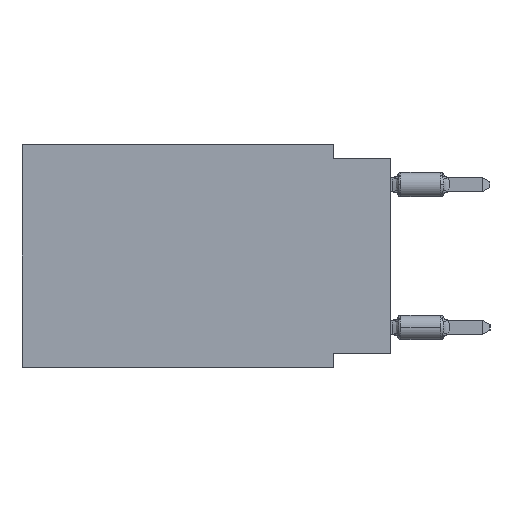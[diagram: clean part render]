
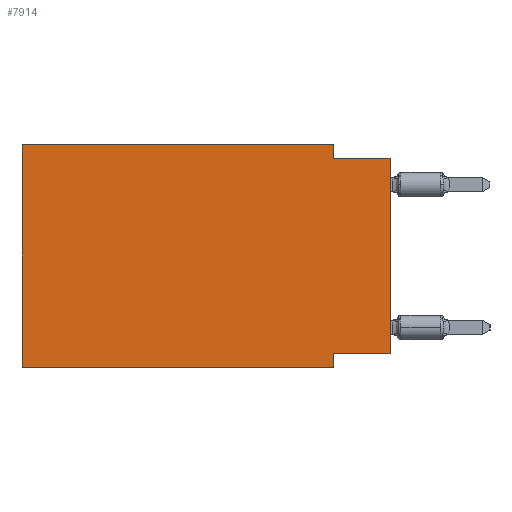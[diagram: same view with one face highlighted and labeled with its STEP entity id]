
A CAD part, left-side view. The second image highlights one B-rep face of the part: STEP entity #7914.
In plain terms, the highlighted planar face has unit normal (-1, 0, 0).
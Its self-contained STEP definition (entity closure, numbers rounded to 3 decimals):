
#79 = VECTOR ( 'NONE', #2542, 1000. ) ;
#182 = CARTESIAN_POINT ( 'NONE',  ( 0., 16.383, -9.906 ) ) ;
#345 = FACE_OUTER_BOUND ( 'NONE', #1507, .T. ) ;
#1161 = DIRECTION ( 'NONE',  ( 0., 1., 0. ) ) ;
#1223 = LINE ( 'NONE', #20597, #79 ) ;
#1426 = AXIS2_PLACEMENT_3D ( 'NONE', #5745, #12348, #20137 ) ;
#1507 = EDGE_LOOP ( 'NONE', ( #10673, #5341, #10723, #15838, #16441, #10533, #19143, #2085 ) ) ;
#1753 = DIRECTION ( 'NONE',  ( 0., -1., 0. ) ) ;
#1975 = VECTOR ( 'NONE', #2917, 1000. ) ;
#2085 = ORIENTED_EDGE ( 'NONE', *, *, #8417, .F. ) ;
#2102 = CARTESIAN_POINT ( 'NONE',  ( 0., 0., 0. ) ) ;
#2542 = DIRECTION ( 'NONE',  ( 0., 0., -1. ) ) ;
#2917 = DIRECTION ( 'NONE',  ( 0., -1., 0. ) ) ;
#3406 = EDGE_CURVE ( 'NONE', #12749, #7236, #16147, .T. ) ;
#4441 = LINE ( 'NONE', #12976, #1975 ) ;
#4716 = LINE ( 'NONE', #182, #6867 ) ;
#5341 = ORIENTED_EDGE ( 'NONE', *, *, #3406, .F. ) ;
#5731 = CARTESIAN_POINT ( 'NONE',  ( 0., 2.54, -9.906 ) ) ;
#5745 = CARTESIAN_POINT ( 'NONE',  ( 0., 16.383, 0. ) ) ;
#6389 = CARTESIAN_POINT ( 'NONE',  ( 0., 2.54, -9.906 ) ) ;
#6755 = VERTEX_POINT ( 'NONE', #16113 ) ;
#6867 = VECTOR ( 'NONE', #13156, 1000. ) ;
#7076 = DIRECTION ( 'NONE',  ( 0., 0., 1. ) ) ;
#7236 = VERTEX_POINT ( 'NONE', #12630 ) ;
#7678 = VECTOR ( 'NONE', #16793, 1000. ) ;
#7914 = ADVANCED_FACE ( 'NONE', ( #345 ), #20558, .F. ) ;
#8417 = EDGE_CURVE ( 'NONE', #15173, #13292, #14359, .T. ) ;
#10195 = EDGE_CURVE ( 'NONE', #6755, #12749, #1223, .T. ) ;
#10277 = LINE ( 'NONE', #5731, #21040 ) ;
#10295 = CARTESIAN_POINT ( 'NONE',  ( 0., 2.54, -9.271 ) ) ;
#10300 = EDGE_CURVE ( 'NONE', #12628, #18626, #13645, .T. ) ;
#10533 = ORIENTED_EDGE ( 'NONE', *, *, #19527, .T. ) ;
#10673 = ORIENTED_EDGE ( 'NONE', *, *, #13018, .T. ) ;
#10723 = ORIENTED_EDGE ( 'NONE', *, *, #10195, .F. ) ;
#10767 = VECTOR ( 'NONE', #7076, 1000. ) ;
#10788 = VECTOR ( 'NONE', #1161, 1000. ) ;
#11514 = CARTESIAN_POINT ( 'NONE',  ( 0., 16.383, 0. ) ) ;
#12348 = DIRECTION ( 'NONE',  ( 1., 0., 0. ) ) ;
#12628 = VERTEX_POINT ( 'NONE', #18678 ) ;
#12630 = CARTESIAN_POINT ( 'NONE',  ( 0., 0., -0.635 ) ) ;
#12749 = VERTEX_POINT ( 'NONE', #16278 ) ;
#12976 = CARTESIAN_POINT ( 'NONE',  ( 0., 16.383, 0. ) ) ;
#13014 = CARTESIAN_POINT ( 'NONE',  ( 0., 16.383, 0. ) ) ;
#13018 = EDGE_CURVE ( 'NONE', #15173, #7236, #17248, .T. ) ;
#13156 = DIRECTION ( 'NONE',  ( 0., -1., 0. ) ) ;
#13292 = VERTEX_POINT ( 'NONE', #10295 ) ;
#13645 = LINE ( 'NONE', #11514, #7678 ) ;
#13850 = DIRECTION ( 'NONE',  ( 0., 0., -1. ) ) ;
#14359 = LINE ( 'NONE', #18919, #10788 ) ;
#15173 = VERTEX_POINT ( 'NONE', #19592 ) ;
#15838 = ORIENTED_EDGE ( 'NONE', *, *, #20787, .F. ) ;
#16113 = CARTESIAN_POINT ( 'NONE',  ( 0., 2.54, 0. ) ) ;
#16147 = LINE ( 'NONE', #17877, #20723 ) ;
#16278 = CARTESIAN_POINT ( 'NONE',  ( 0., 2.54, -0.635 ) ) ;
#16441 = ORIENTED_EDGE ( 'NONE', *, *, #10300, .F. ) ;
#16793 = DIRECTION ( 'NONE',  ( 0., 0., 1. ) ) ;
#17248 = LINE ( 'NONE', #2102, #10767 ) ;
#17614 = EDGE_CURVE ( 'NONE', #13292, #19109, #10277, .T. ) ;
#17877 = CARTESIAN_POINT ( 'NONE',  ( 0., 0., -0.635 ) ) ;
#18626 = VERTEX_POINT ( 'NONE', #13014 ) ;
#18678 = CARTESIAN_POINT ( 'NONE',  ( 0., 16.383, -9.906 ) ) ;
#18919 = CARTESIAN_POINT ( 'NONE',  ( 0., 0., -9.271 ) ) ;
#19109 = VERTEX_POINT ( 'NONE', #6389 ) ;
#19143 = ORIENTED_EDGE ( 'NONE', *, *, #17614, .F. ) ;
#19527 = EDGE_CURVE ( 'NONE', #12628, #19109, #4716, .T. ) ;
#19592 = CARTESIAN_POINT ( 'NONE',  ( 0., 0., -9.271 ) ) ;
#20137 = DIRECTION ( 'NONE',  ( 0., 0., -1. ) ) ;
#20558 = PLANE ( 'NONE',  #1426 ) ;
#20597 = CARTESIAN_POINT ( 'NONE',  ( 0., 2.54, 0. ) ) ;
#20723 = VECTOR ( 'NONE', #1753, 1000. ) ;
#20787 = EDGE_CURVE ( 'NONE', #18626, #6755, #4441, .T. ) ;
#21040 = VECTOR ( 'NONE', #13850, 1000. ) ;
